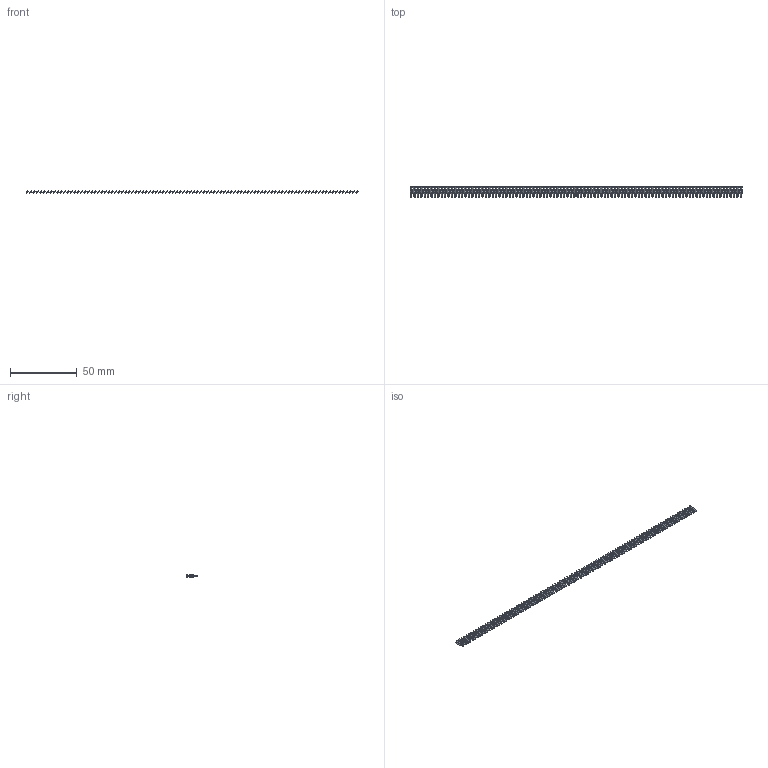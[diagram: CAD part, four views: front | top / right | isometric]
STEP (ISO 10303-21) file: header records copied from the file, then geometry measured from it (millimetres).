
FILE_DESCRIPTION (( 'STEP AP203' ), '1' );
FILE_NAME ('106-098-253-100.STEP', '2020-04-16T23:09:13', ( '' ), ( '' ), 'SwSTEP 2.0', 'SolidWorks 2016', '' );
FILE_SCHEMA (( 'CONFIG_CONTROL_DESIGN' ));
Length unit declared in the file: inch
Products named in the file (2): 106-098-253-100; 100-290-001_100-290-253
Assembly tree (98 placements, depth 2):
  106-098-253-100
    100-290-001_100-290-253  x98
Bounding box: 248.18 x 7.62 x 1.8 mm (x, y, z)
Volume: 540.7 mm3; surface area: 3371.9 mm2
Topology: 98 solids, 98 shells, 1960 faces, 5292 edges, 3528 vertices
Faces by surface type: plane 1862, cylinder 98
Entity records: 3924 total; most frequent: DIRECTION 298, CARTESIAN_POINT 211, DATE_AND_TIME 206, COORDINATED_UNIVERSAL_TIME_OFFSET 206, CALENDAR_DATE 206, LOCAL_TIME 206, AXIS2_PLACEMENT_3D 123, PERSON_AND_ORGANIZATION 114
